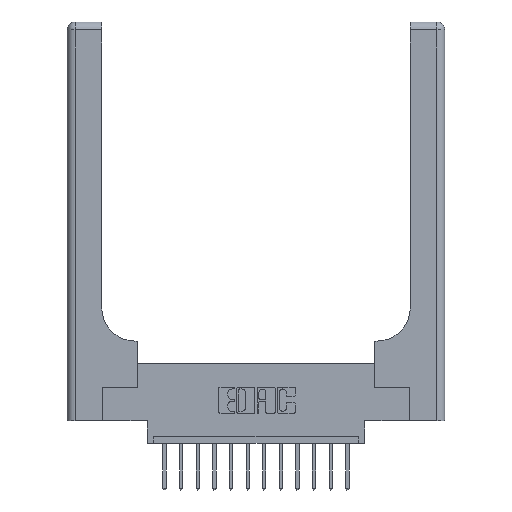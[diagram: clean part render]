
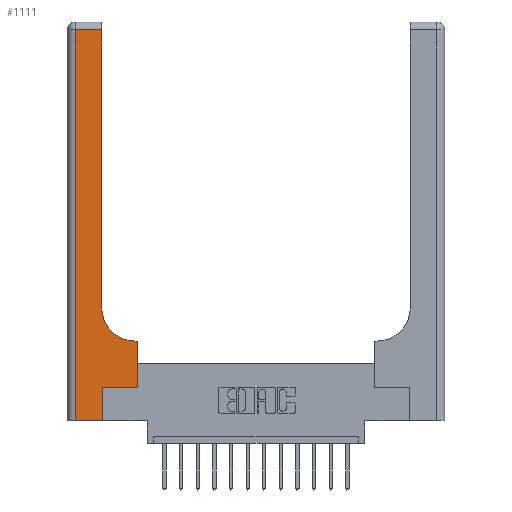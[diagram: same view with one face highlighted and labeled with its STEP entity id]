
A CAD part, top view. The second image highlights one B-rep face of the part: STEP entity #1111.
In plain terms, the highlighted planar face has unit normal (0, 0, 1).
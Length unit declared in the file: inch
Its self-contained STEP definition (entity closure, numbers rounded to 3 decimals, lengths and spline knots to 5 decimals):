
#62 = DIRECTION ( 'NONE',  ( -1., 0., 0. ) ) ;
#68 = CIRCLE ( 'NONE', #16219, 0.25 ) ;
#102 = LINE ( 'NONE', #2981, #11134 ) ;
#471 = VERTEX_POINT ( 'NONE', #8900 ) ;
#935 = CARTESIAN_POINT ( 'NONE',  ( 0.26, 3., 0.37 ) ) ;
#1111 = ADVANCED_FACE ( 'NONE', ( #13336 ), #14361, .F. ) ;
#1120 = VERTEX_POINT ( 'NONE', #7925 ) ;
#1213 = CARTESIAN_POINT ( 'NONE',  ( 0., 3., 0.37 ) ) ;
#1382 = DIRECTION ( 'NONE',  ( 0., 0., -1. ) ) ;
#1829 = EDGE_CURVE ( 'NONE', #471, #2943, #1972, .T. ) ;
#1972 = LINE ( 'NONE', #6001, #15864 ) ;
#2016 = EDGE_CURVE ( 'NONE', #1120, #8563, #102, .T. ) ;
#2372 = CARTESIAN_POINT ( 'NONE',  ( 0.51, 0.85, 0.37 ) ) ;
#2603 = VERTEX_POINT ( 'NONE', #11611 ) ;
#2604 = VECTOR ( 'NONE', #16761, 39.37008 ) ;
#2636 = EDGE_LOOP ( 'NONE', ( #13865, #10808, #17248, #6286, #4005, #15774, #2683, #13798, #13799 ) ) ;
#2679 = VECTOR ( 'NONE', #10046, 39.37008 ) ;
#2683 = ORIENTED_EDGE ( 'NONE', *, *, #1829, .T. ) ;
#2943 = VERTEX_POINT ( 'NONE', #9926 ) ;
#2981 = CARTESIAN_POINT ( 'NONE',  ( 0., 2.94, 0.37 ) ) ;
#3735 = LINE ( 'NONE', #11534, #8500 ) ;
#3774 = EDGE_CURVE ( 'NONE', #14098, #2603, #68, .T. ) ;
#3971 = VERTEX_POINT ( 'NONE', #5850 ) ;
#4005 = ORIENTED_EDGE ( 'NONE', *, *, #5984, .T. ) ;
#4270 = VECTOR ( 'NONE', #9938, 39.37008 ) ;
#4303 = DIRECTION ( 'NONE',  ( -1., 0., 0. ) ) ;
#5309 = EDGE_CURVE ( 'NONE', #9919, #471, #3735, .T. ) ;
#5477 = CARTESIAN_POINT ( 'NONE',  ( 0.265, 0.25, 0.37 ) ) ;
#5675 = LINE ( 'NONE', #935, #4270 ) ;
#5792 = CARTESIAN_POINT ( 'NONE',  ( 0.06, 2.94, 0.37 ) ) ;
#5850 = CARTESIAN_POINT ( 'NONE',  ( 0.265, 0., 0.37 ) ) ;
#5984 = EDGE_CURVE ( 'NONE', #3971, #9919, #15998, .T. ) ;
#6001 = CARTESIAN_POINT ( 'NONE',  ( 0.528, 0.25, 0.37 ) ) ;
#6286 = ORIENTED_EDGE ( 'NONE', *, *, #14955, .T. ) ;
#6298 = DIRECTION ( 'NONE',  ( 1., 0., 0. ) ) ;
#7419 = CARTESIAN_POINT ( 'NONE',  ( 0., 0., 0.37 ) ) ;
#7509 = VECTOR ( 'NONE', #16827, 39.37008 ) ;
#7691 = DIRECTION ( 'NONE',  ( 0., 0., -1. ) ) ;
#7925 = CARTESIAN_POINT ( 'NONE',  ( 0.26, 2.94, 0.37 ) ) ;
#8500 = VECTOR ( 'NONE', #6298, 39.37008 ) ;
#8563 = VERTEX_POINT ( 'NONE', #5792 ) ;
#8648 = LINE ( 'NONE', #11543, #7509 ) ;
#8764 = CARTESIAN_POINT ( 'NONE',  ( 0.06, 3., 0.37 ) ) ;
#8822 = EDGE_CURVE ( 'NONE', #2603, #1120, #5675, .T. ) ;
#8900 = CARTESIAN_POINT ( 'NONE',  ( 0.528, 0.25, 0.37 ) ) ;
#9770 = VERTEX_POINT ( 'NONE', #11703 ) ;
#9919 = VERTEX_POINT ( 'NONE', #5477 ) ;
#9926 = CARTESIAN_POINT ( 'NONE',  ( 0.528, 0.6, 0.37 ) ) ;
#9938 = DIRECTION ( 'NONE',  ( 0., 1., 0. ) ) ;
#10046 = DIRECTION ( 'NONE',  ( 1., 0., 0. ) ) ;
#10068 = LINE ( 'NONE', #8764, #2604 ) ;
#10090 = CARTESIAN_POINT ( 'NONE',  ( 0.51, 0.6, 0.37 ) ) ;
#10773 = VECTOR ( 'NONE', #15115, 39.37008 ) ;
#10808 = ORIENTED_EDGE ( 'NONE', *, *, #2016, .T. ) ;
#11134 = VECTOR ( 'NONE', #4303, 39.37008 ) ;
#11534 = CARTESIAN_POINT ( 'NONE',  ( 0.265, 0.25, 0.37 ) ) ;
#11543 = CARTESIAN_POINT ( 'NONE',  ( 0.26, 0.6, 0.37 ) ) ;
#11611 = CARTESIAN_POINT ( 'NONE',  ( 0.26, 0.85, 0.37 ) ) ;
#11703 = CARTESIAN_POINT ( 'NONE',  ( 0.06, 0., 0.37 ) ) ;
#11728 = DIRECTION ( 'NONE',  ( 1., 0., 0. ) ) ;
#12503 = LINE ( 'NONE', #7419, #2679 ) ;
#12555 = AXIS2_PLACEMENT_3D ( 'NONE', #1213, #1382, #62 ) ;
#12586 = EDGE_CURVE ( 'NONE', #2943, #14098, #8648, .T. ) ;
#13336 = FACE_OUTER_BOUND ( 'NONE', #2636, .T. ) ;
#13488 = CARTESIAN_POINT ( 'NONE',  ( 0.265, 0., 0.37 ) ) ;
#13798 = ORIENTED_EDGE ( 'NONE', *, *, #12586, .T. ) ;
#13799 = ORIENTED_EDGE ( 'NONE', *, *, #3774, .T. ) ;
#13865 = ORIENTED_EDGE ( 'NONE', *, *, #8822, .T. ) ;
#14098 = VERTEX_POINT ( 'NONE', #10090 ) ;
#14361 = PLANE ( 'NONE',  #12555 ) ;
#14528 = EDGE_CURVE ( 'NONE', #8563, #9770, #10068, .T. ) ;
#14955 = EDGE_CURVE ( 'NONE', #9770, #3971, #12503, .T. ) ;
#15115 = DIRECTION ( 'NONE',  ( 0., 1., 0. ) ) ;
#15774 = ORIENTED_EDGE ( 'NONE', *, *, #5309, .T. ) ;
#15864 = VECTOR ( 'NONE', #16599, 39.37008 ) ;
#15998 = LINE ( 'NONE', #13488, #10773 ) ;
#16219 = AXIS2_PLACEMENT_3D ( 'NONE', #2372, #7691, #11728 ) ;
#16599 = DIRECTION ( 'NONE',  ( 0., 1., 0. ) ) ;
#16761 = DIRECTION ( 'NONE',  ( 0., -1., 0. ) ) ;
#16827 = DIRECTION ( 'NONE',  ( -1., 0., 0. ) ) ;
#17248 = ORIENTED_EDGE ( 'NONE', *, *, #14528, .T. ) ;
